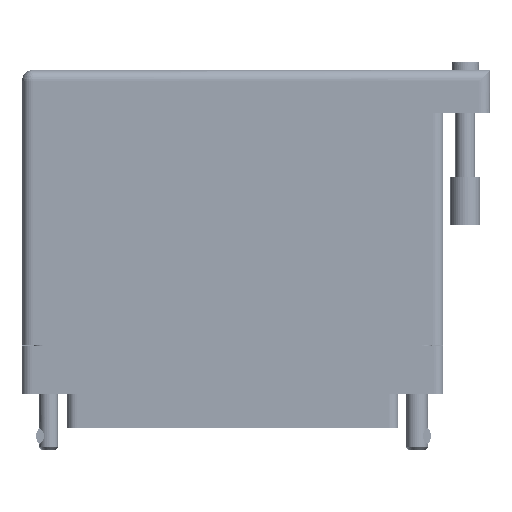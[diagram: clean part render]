
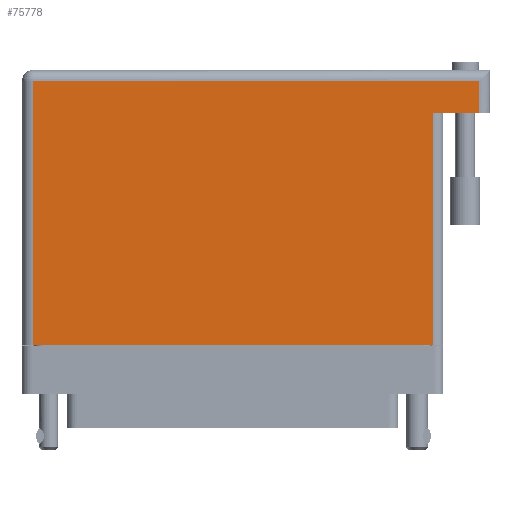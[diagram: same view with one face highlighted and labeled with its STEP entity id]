
A CAD part, front view. The second image highlights one B-rep face of the part: STEP entity #75778.
In plain terms, the highlighted face is planar.
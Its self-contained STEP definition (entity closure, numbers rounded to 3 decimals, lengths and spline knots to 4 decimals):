
#587 = CARTESIAN_POINT ( 'NONE',  ( -1.289, -0.1, 0.617 ) ) ;
#1621 = CARTESIAN_POINT ( 'NONE',  ( -1.289, -0.1, 0.617 ) ) ;
#2935 = ORIENTED_EDGE ( 'NONE', *, *, #52011, .T. ) ;
#3997 = VERTEX_POINT ( 'NONE', #42756 ) ;
#4129 = DIRECTION ( 'NONE',  ( 0., 0., -1. ) ) ;
#5426 = DIRECTION ( 'NONE',  ( 0., 1., 0. ) ) ;
#5714 = CARTESIAN_POINT ( 'NONE',  ( 1.289, 1.395, 0.617 ) ) ;
#6868 = LINE ( 'NONE', #5714, #73669 ) ;
#6996 = CARTESIAN_POINT ( 'NONE',  ( -1.289, 1.605, 0.617 ) ) ;
#13643 = LINE ( 'NONE', #55959, #75415 ) ;
#14144 = EDGE_CURVE ( 'NONE', #50144, #29693, #54850, .T. ) ;
#15368 = EDGE_CURVE ( 'NONE', #29693, #51775, #47480, .T. ) ;
#15393 = FACE_OUTER_BOUND ( 'NONE', #33491, .T. ) ;
#16658 = CARTESIAN_POINT ( 'NONE',  ( -1.359, 1.605, 0.617 ) ) ;
#20671 = ORIENTED_EDGE ( 'NONE', *, *, #14144, .T. ) ;
#23027 = ORIENTED_EDGE ( 'NONE', *, *, #24974, .F. ) ;
#23552 = LINE ( 'NONE', #69476, #52834 ) ;
#23714 = PLANE ( 'NONE',  #43874 ) ;
#24974 = EDGE_CURVE ( 'NONE', #69588, #51029, #23552, .T. ) ;
#25328 = VECTOR ( 'NONE', #42782, 39.3701 ) ;
#25998 = LINE ( 'NONE', #16658, #40139 ) ;
#26175 = ORIENTED_EDGE ( 'NONE', *, *, #47900, .T. ) ;
#29693 = VERTEX_POINT ( 'NONE', #1621 ) ;
#33491 = EDGE_LOOP ( 'NONE', ( #55904, #2935, #23027, #69932, #26175, #20671 ) ) ;
#36997 = DIRECTION ( 'NONE',  ( -1., 0., 0. ) ) ;
#40139 = VECTOR ( 'NONE', #56526, 39.3701 ) ;
#42756 = CARTESIAN_POINT ( 'NONE',  ( 1.589, 1.605, 0.617 ) ) ;
#42782 = DIRECTION ( 'NONE',  ( 1., 0., 0. ) ) ;
#43874 = AXIS2_PLACEMENT_3D ( 'NONE', #69500, #4129, #36997 ) ;
#44802 = DIRECTION ( 'NONE',  ( -1., 0., 0. ) ) ;
#47480 = LINE ( 'NONE', #54993, #25328 ) ;
#47900 = EDGE_CURVE ( 'NONE', #3997, #50144, #25998, .T. ) ;
#48824 = DIRECTION ( 'NONE',  ( 0., 1., 0. ) ) ;
#50144 = VERTEX_POINT ( 'NONE', #6996 ) ;
#51029 = VERTEX_POINT ( 'NONE', #70071 ) ;
#51775 = VERTEX_POINT ( 'NONE', #77858 ) ;
#52011 = EDGE_CURVE ( 'NONE', #51775, #51029, #6868, .T. ) ;
#52834 = VECTOR ( 'NONE', #44802, 39.3701 ) ;
#54553 = EDGE_CURVE ( 'NONE', #69588, #3997, #13643, .T. ) ;
#54850 = LINE ( 'NONE', #587, #57806 ) ;
#54993 = CARTESIAN_POINT ( 'NONE',  ( -1.359, -0.1, 0.617 ) ) ;
#55904 = ORIENTED_EDGE ( 'NONE', *, *, #15368, .T. ) ;
#55959 = CARTESIAN_POINT ( 'NONE',  ( 1.589, 1.675, 0.617 ) ) ;
#56526 = DIRECTION ( 'NONE',  ( -1., 0., 0. ) ) ;
#57806 = VECTOR ( 'NONE', #77519, 39.3701 ) ;
#69476 = CARTESIAN_POINT ( 'NONE',  ( 1.659, 1.395, 0.617 ) ) ;
#69500 = CARTESIAN_POINT ( 'NONE',  ( -1.359, 1.675, 0.617 ) ) ;
#69588 = VERTEX_POINT ( 'NONE', #75988 ) ;
#69932 = ORIENTED_EDGE ( 'NONE', *, *, #54553, .T. ) ;
#70071 = CARTESIAN_POINT ( 'NONE',  ( 1.289, 1.395, 0.617 ) ) ;
#73669 = VECTOR ( 'NONE', #5426, 39.3701 ) ;
#75415 = VECTOR ( 'NONE', #48824, 39.3701 ) ;
#75778 = ADVANCED_FACE ( 'NONE', ( #15393 ), #23714, .F. ) ;
#75988 = CARTESIAN_POINT ( 'NONE',  ( 1.589, 1.395, 0.617 ) ) ;
#77519 = DIRECTION ( 'NONE',  ( 0., -1., 0. ) ) ;
#77858 = CARTESIAN_POINT ( 'NONE',  ( 1.289, -0.1, 0.617 ) ) ;
